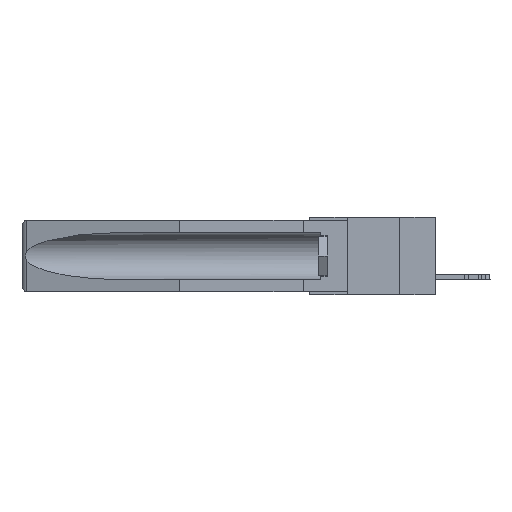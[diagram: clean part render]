
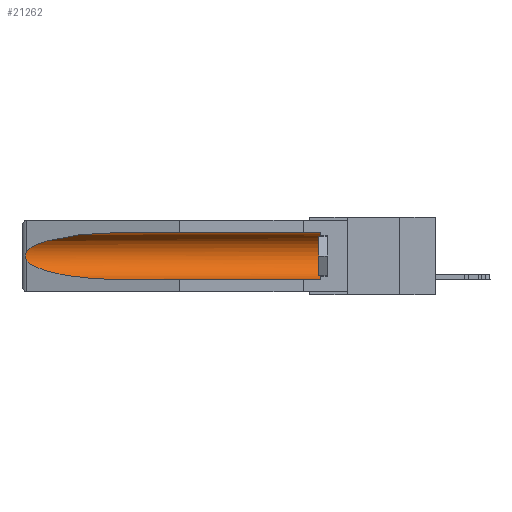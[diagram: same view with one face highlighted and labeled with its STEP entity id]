
A CAD part, left-side view. The second image highlights one B-rep face of the part: STEP entity #21262.
In plain terms, the highlighted cylindrical face has radius 2.857 mm (diameter 5.715 mm), a partial arc.
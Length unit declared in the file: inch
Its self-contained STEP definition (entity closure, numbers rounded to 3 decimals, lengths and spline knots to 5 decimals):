
#109 =( BOUNDED_CURVE ( )  B_SPLINE_CURVE ( 3, ( #27101, #10400, #569, #783 ),
 .UNSPECIFIED., .F., .F. ) 
 B_SPLINE_CURVE_WITH_KNOTS ( ( 4, 4 ),
 ( 4.71239, 6.08839 ),
 .UNSPECIFIED. ) 
 CURVE ( )  GEOMETRIC_REPRESENTATION_ITEM ( )  RATIONAL_B_SPLINE_CURVE ( ( 1., 0.848, 0.848, 1. ) ) 
 REPRESENTATION_ITEM ( '' )  );
#569 = CARTESIAN_POINT ( 'NONE',  ( 0.25451, 1.48313, -0.09465 ) ) ;
#783 = CARTESIAN_POINT ( 'NONE',  ( 0.26537, 1.52718, -0.14972 ) ) ;
#946 = CARTESIAN_POINT ( 'NONE',  ( 0.26597, 1.52961, -0.15275 ) ) ;
#1842 = CYLINDRICAL_SURFACE ( 'NONE', #17794, 0.1125 ) ;
#2309 = CARTESIAN_POINT ( 'NONE',  ( 0.155, 0.126, -0.1715 ) ) ;
#3203 = CARTESIAN_POINT ( 'NONE',  ( 0.2673, 1.5327, -0.16383 ) ) ;
#3554 = CARTESIAN_POINT ( 'NONE',  ( 0.155, -0.30754, -0.1715 ) ) ;
#4168 = CARTESIAN_POINT ( 'NONE',  ( 0.155, 0.126, -0.059 ) ) ;
#4397 = LINE ( 'NONE', #26472, #15716 ) ;
#4745 = DIRECTION ( 'NONE',  ( 0., 1., 0. ) ) ;
#4848 = VECTOR ( 'NONE', #8151, 39.37008 ) ;
#4856 = EDGE_CURVE ( 'NONE', #29426, #5365, #28739, .T. ) ;
#5160 = DIRECTION ( 'NONE',  ( 0., -1., 0. ) ) ;
#5365 = VERTEX_POINT ( 'NONE', #18119 ) ;
#6030 = CARTESIAN_POINT ( 'NONE',  ( 0.155, -0.30754, -0.284 ) ) ;
#7223 = VERTEX_POINT ( 'NONE', #12113 ) ;
#7982 = CARTESIAN_POINT ( 'NONE',  ( 0.26597, 1.5296, -0.19026 ) ) ;
#8151 = DIRECTION ( 'NONE',  ( 0., 1., 0. ) ) ;
#8837 = EDGE_CURVE ( 'NONE', #12811, #29232, #23358, .T. ) ;
#9255 = ORIENTED_EDGE ( 'NONE', *, *, #4856, .T. ) ;
#10400 = CARTESIAN_POINT ( 'NONE',  ( 0.21114, 1.30732, -0.059 ) ) ;
#10678 = CARTESIAN_POINT ( 'NONE',  ( 0.2673, 1.53269, -0.17917 ) ) ;
#11857 = ORIENTED_EDGE ( 'NONE', *, *, #24099, .T. ) ;
#12113 = CARTESIAN_POINT ( 'NONE',  ( 0.155, 1.07973, -0.059 ) ) ;
#12392 = ORIENTED_EDGE ( 'NONE', *, *, #8837, .F. ) ;
#12811 = VERTEX_POINT ( 'NONE', #31035 ) ;
#15716 = VECTOR ( 'NONE', #4745, 39.37008 ) ;
#15949 = CARTESIAN_POINT ( 'NONE',  ( 0.26537, 1.52718, -0.14972 ) ) ;
#16627 = ORIENTED_EDGE ( 'NONE', *, *, #20550, .T. ) ;
#17044 = ORIENTED_EDGE ( 'NONE', *, *, #25327, .T. ) ;
#17794 = AXIS2_PLACEMENT_3D ( 'NONE', #3554, #23201, #27814 ) ;
#17873 = CARTESIAN_POINT ( 'NONE',  ( 0.26655, 1.53094, -0.18657 ) ) ;
#17969 = CARTESIAN_POINT ( 'NONE',  ( 0.2675, 1.53308, -0.17534 ) ) ;
#18119 = CARTESIAN_POINT ( 'NONE',  ( 0.26537, 1.52718, -0.19328 ) ) ;
#19011 = CARTESIAN_POINT ( 'NONE',  ( 0.21114, 1.30732, -0.284 ) ) ;
#19120 = CARTESIAN_POINT ( 'NONE',  ( 0.155, 1.07973, -0.284 ) ) ;
#19599 = DIRECTION ( 'NONE',  ( 0., 0., 1. ) ) ;
#19834 = AXIS2_PLACEMENT_3D ( 'NONE', #2309, #5160, #19599 ) ;
#20550 = EDGE_CURVE ( 'NONE', #7223, #29426, #109, .T. ) ;
#21110 = CARTESIAN_POINT ( 'NONE',  ( 0.26537, 1.52718, -0.19328 ) ) ;
#21262 = ADVANCED_FACE ( 'NONE', ( #31298 ), #1842, .F. ) ;
#22513 = EDGE_CURVE ( 'NONE', #12811, #26699, #30592, .T. ) ;
#23201 = DIRECTION ( 'NONE',  ( 0., 1., 0. ) ) ;
#23358 = LINE ( 'NONE', #6030, #4848 ) ;
#24099 = EDGE_CURVE ( 'NONE', #5365, #29232, #25864, .T. ) ;
#24641 = CARTESIAN_POINT ( 'NONE',  ( 0.155, 1.07973, -0.284 ) ) ;
#24952 = CARTESIAN_POINT ( 'NONE',  ( 0.26537, 1.52718, -0.19328 ) ) ;
#25145 = CARTESIAN_POINT ( 'NONE',  ( 0.26537, 1.52718, -0.14972 ) ) ;
#25327 = EDGE_CURVE ( 'NONE', #26699, #7223, #4397, .T. ) ;
#25864 =( BOUNDED_CURVE ( )  B_SPLINE_CURVE ( 3, ( #21110, #26194, #19011, #19120 ),
 .UNSPECIFIED., .F., .F. ) 
 B_SPLINE_CURVE_WITH_KNOTS ( ( 4, 4 ),
 ( 0.1948, 1.5708 ),
 .UNSPECIFIED. ) 
 CURVE ( )  GEOMETRIC_REPRESENTATION_ITEM ( )  RATIONAL_B_SPLINE_CURVE ( ( 1., 0.848, 0.848, 1. ) ) 
 REPRESENTATION_ITEM ( '' )  );
#26194 = CARTESIAN_POINT ( 'NONE',  ( 0.25451, 1.48313, -0.24835 ) ) ;
#26472 = CARTESIAN_POINT ( 'NONE',  ( 0.155, -0.30754, -0.059 ) ) ;
#26699 = VERTEX_POINT ( 'NONE', #4168 ) ;
#26863 = ORIENTED_EDGE ( 'NONE', *, *, #22513, .T. ) ;
#27101 = CARTESIAN_POINT ( 'NONE',  ( 0.155, 1.07973, -0.059 ) ) ;
#27814 = DIRECTION ( 'NONE',  ( 0., 0., 1. ) ) ;
#28739 = B_SPLINE_CURVE_WITH_KNOTS ( 'NONE', 3,
 ( #25145, #946, #29647, #3203, #30073, #17969, #10678, #17873, #7982, #24952 ),
 .UNSPECIFIED., .F., .F.,
 ( 4, 2, 2, 2, 4 ),
 ( 0., 0.00029, 0.00058, 0.00087, 0.00117 ),
 .UNSPECIFIED. ) ;
#29232 = VERTEX_POINT ( 'NONE', #24641 ) ;
#29426 = VERTEX_POINT ( 'NONE', #15949 ) ;
#29647 = CARTESIAN_POINT ( 'NONE',  ( 0.26654, 1.53092, -0.15636 ) ) ;
#30073 = CARTESIAN_POINT ( 'NONE',  ( 0.2675, 1.53308, -0.16763 ) ) ;
#30592 = CIRCLE ( 'NONE', #19834, 0.1125 ) ;
#30898 = EDGE_LOOP ( 'NONE', ( #16627, #9255, #11857, #12392, #26863, #17044 ) ) ;
#31035 = CARTESIAN_POINT ( 'NONE',  ( 0.155, 0.126, -0.284 ) ) ;
#31298 = FACE_OUTER_BOUND ( 'NONE', #30898, .T. ) ;
